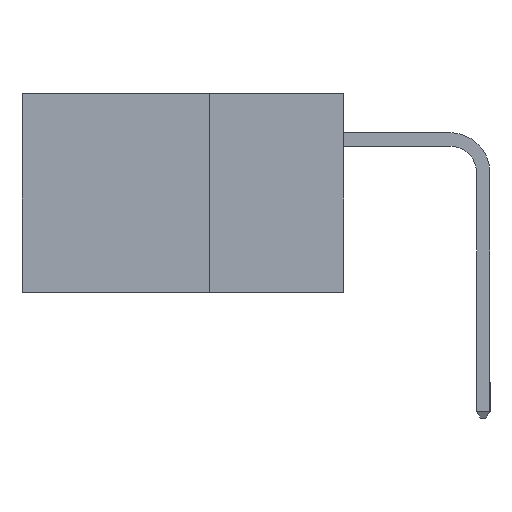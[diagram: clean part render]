
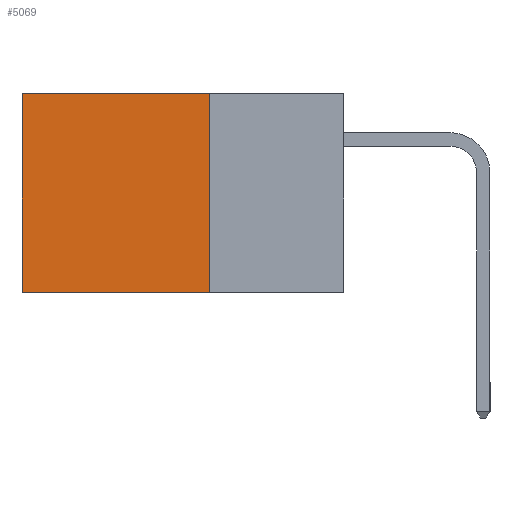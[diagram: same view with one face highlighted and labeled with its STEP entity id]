
A CAD part, left-side view. The second image highlights one B-rep face of the part: STEP entity #5069.
In plain terms, the highlighted planar face has unit normal (-1, 0, 0).
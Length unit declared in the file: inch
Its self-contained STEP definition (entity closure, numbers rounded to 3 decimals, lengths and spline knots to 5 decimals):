
#288 = CARTESIAN_POINT ( 'NONE',  ( 0.298, 0.25, 0. ) ) ;
#616 = EDGE_LOOP ( 'NONE', ( #6694, #4327, #1758, #10065 ) ) ;
#760 = DIRECTION ( 'NONE',  ( 0., 1., 0. ) ) ;
#832 = EDGE_CURVE ( 'NONE', #2032, #3827, #8347, .T. ) ;
#1193 = VECTOR ( 'NONE', #760, 39.37008 ) ;
#1489 = LINE ( 'NONE', #3692, #6016 ) ;
#1619 = DIRECTION ( 'NONE',  ( 0., 0., -1. ) ) ;
#1636 = DIRECTION ( 'NONE',  ( 1., 0., 0. ) ) ;
#1758 = ORIENTED_EDGE ( 'NONE', *, *, #8951, .F. ) ;
#2032 = VERTEX_POINT ( 'NONE', #4976 ) ;
#2337 = LINE ( 'NONE', #6360, #11374 ) ;
#2849 = PLANE ( 'NONE',  #8117 ) ;
#3260 = EDGE_CURVE ( 'NONE', #3827, #5451, #11088, .T. ) ;
#3572 = DIRECTION ( 'NONE',  ( 0., 1., 0. ) ) ;
#3692 = CARTESIAN_POINT ( 'NONE',  ( 0.298, 0.25, -0.37 ) ) ;
#3827 = VERTEX_POINT ( 'NONE', #4679 ) ;
#4018 = FACE_OUTER_BOUND ( 'NONE', #616, .T. ) ;
#4316 = CARTESIAN_POINT ( 'NONE',  ( 0.298, 0.25, 0. ) ) ;
#4327 = ORIENTED_EDGE ( 'NONE', *, *, #7309, .F. ) ;
#4679 = CARTESIAN_POINT ( 'NONE',  ( 0.298, 0.6, 0. ) ) ;
#4976 = CARTESIAN_POINT ( 'NONE',  ( 0.298, 0.25, 0. ) ) ;
#5069 = ADVANCED_FACE ( 'NONE', ( #4018 ), #2849, .F. ) ;
#5451 = VERTEX_POINT ( 'NONE', #10691 ) ;
#6016 = VECTOR ( 'NONE', #3572, 39.37008 ) ;
#6360 = CARTESIAN_POINT ( 'NONE',  ( 0.298, 0.25, 0. ) ) ;
#6694 = ORIENTED_EDGE ( 'NONE', *, *, #3260, .T. ) ;
#6724 = CARTESIAN_POINT ( 'NONE',  ( 0.298, 0.25, -0.37 ) ) ;
#7309 = EDGE_CURVE ( 'NONE', #10582, #5451, #1489, .T. ) ;
#8117 = AXIS2_PLACEMENT_3D ( 'NONE', #288, #1636, #1619 ) ;
#8347 = LINE ( 'NONE', #4316, #1193 ) ;
#8777 = VECTOR ( 'NONE', #10327, 39.37008 ) ;
#8933 = DIRECTION ( 'NONE',  ( 0., 0., -1. ) ) ;
#8951 = EDGE_CURVE ( 'NONE', #2032, #10582, #2337, .T. ) ;
#9760 = CARTESIAN_POINT ( 'NONE',  ( 0.298, 0.6, 0. ) ) ;
#10065 = ORIENTED_EDGE ( 'NONE', *, *, #832, .T. ) ;
#10327 = DIRECTION ( 'NONE',  ( 0., 0., -1. ) ) ;
#10582 = VERTEX_POINT ( 'NONE', #6724 ) ;
#10691 = CARTESIAN_POINT ( 'NONE',  ( 0.298, 0.6, -0.37 ) ) ;
#11088 = LINE ( 'NONE', #9760, #8777 ) ;
#11374 = VECTOR ( 'NONE', #8933, 39.37008 ) ;
